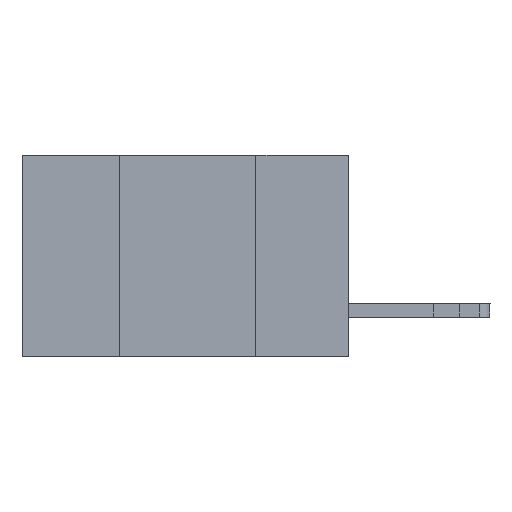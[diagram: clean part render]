
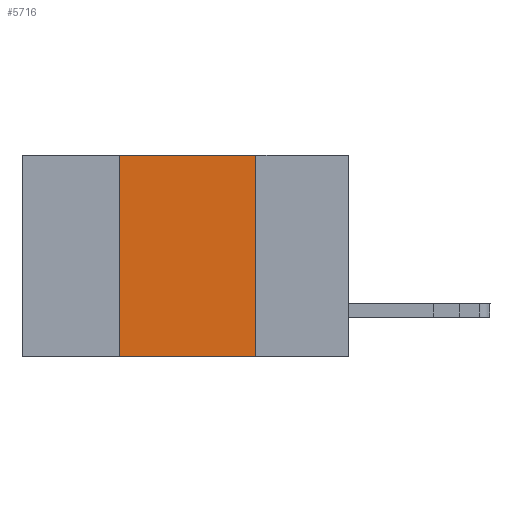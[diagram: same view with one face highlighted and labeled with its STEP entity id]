
A CAD part, left-side view. The second image highlights one B-rep face of the part: STEP entity #5716.
In plain terms, the highlighted planar face has unit normal (-1, 0, 0).
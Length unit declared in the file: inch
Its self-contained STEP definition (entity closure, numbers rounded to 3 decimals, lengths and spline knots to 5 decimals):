
#2 = AXIS2_PLACEMENT_3D ( 'NONE', #10639, #5830, #8238 ) ;
#149 = VECTOR ( 'NONE', #7234, 39.37008 ) ;
#415 = CARTESIAN_POINT ( 'NONE',  ( 0., 0.42, 0. ) ) ;
#725 = VECTOR ( 'NONE', #6430, 39.37008 ) ;
#941 = ORIENTED_EDGE ( 'NONE', *, *, #4583, .F. ) ;
#1533 = EDGE_LOOP ( 'NONE', ( #7475, #6018, #941, #5133 ) ) ;
#2331 = VECTOR ( 'NONE', #13943, 39.37008 ) ;
#2434 = EDGE_CURVE ( 'NONE', #6288, #8825, #10720, .T. ) ;
#4187 = VERTEX_POINT ( 'NONE', #415 ) ;
#4583 = EDGE_CURVE ( 'NONE', #11156, #4187, #13821, .T. ) ;
#4643 = CARTESIAN_POINT ( 'NONE',  ( 0., 0.17, 0. ) ) ;
#5133 = ORIENTED_EDGE ( 'NONE', *, *, #8075, .T. ) ;
#5594 = LINE ( 'NONE', #8082, #10913 ) ;
#5711 = CARTESIAN_POINT ( 'NONE',  ( 0., 0.6, -0.37 ) ) ;
#5716 = ADVANCED_FACE ( 'NONE', ( #12970 ), #15215, .F. ) ;
#5830 = DIRECTION ( 'NONE',  ( 1., 0., 0. ) ) ;
#6018 = ORIENTED_EDGE ( 'NONE', *, *, #14771, .F. ) ;
#6288 = VERTEX_POINT ( 'NONE', #4643 ) ;
#6430 = DIRECTION ( 'NONE',  ( 0., 0., 1. ) ) ;
#7106 = CARTESIAN_POINT ( 'NONE',  ( 0., 0.42, -0.37 ) ) ;
#7234 = DIRECTION ( 'NONE',  ( 0., 0., -1. ) ) ;
#7475 = ORIENTED_EDGE ( 'NONE', *, *, #2434, .F. ) ;
#7924 = CARTESIAN_POINT ( 'NONE',  ( 0., 0.42, 0. ) ) ;
#8075 = EDGE_CURVE ( 'NONE', #11156, #8825, #12777, .T. ) ;
#8082 = CARTESIAN_POINT ( 'NONE',  ( 0., 0.6, 0. ) ) ;
#8238 = DIRECTION ( 'NONE',  ( 0., 0., -1. ) ) ;
#8825 = VERTEX_POINT ( 'NONE', #13374 ) ;
#10639 = CARTESIAN_POINT ( 'NONE',  ( 0., 0.6, 0. ) ) ;
#10720 = LINE ( 'NONE', #14363, #149 ) ;
#10913 = VECTOR ( 'NONE', #12514, 39.37008 ) ;
#11156 = VERTEX_POINT ( 'NONE', #7106 ) ;
#12514 = DIRECTION ( 'NONE',  ( 0., -1., 0. ) ) ;
#12777 = LINE ( 'NONE', #5711, #2331 ) ;
#12970 = FACE_OUTER_BOUND ( 'NONE', #1533, .T. ) ;
#13374 = CARTESIAN_POINT ( 'NONE',  ( 0., 0.17, -0.37 ) ) ;
#13821 = LINE ( 'NONE', #7924, #725 ) ;
#13943 = DIRECTION ( 'NONE',  ( 0., -1., 0. ) ) ;
#14363 = CARTESIAN_POINT ( 'NONE',  ( 0., 0.17, 0. ) ) ;
#14771 = EDGE_CURVE ( 'NONE', #4187, #6288, #5594, .T. ) ;
#15215 = PLANE ( 'NONE',  #2 ) ;
